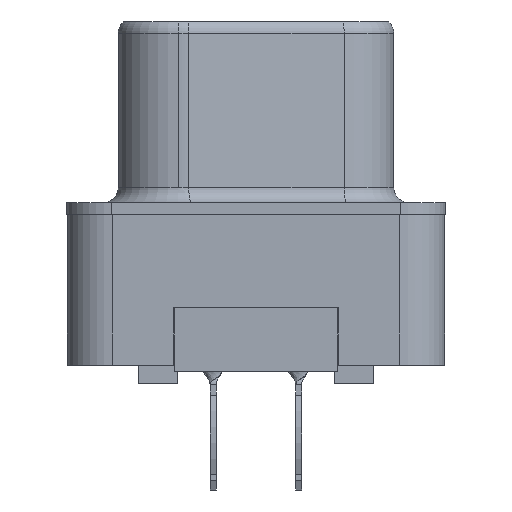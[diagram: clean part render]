
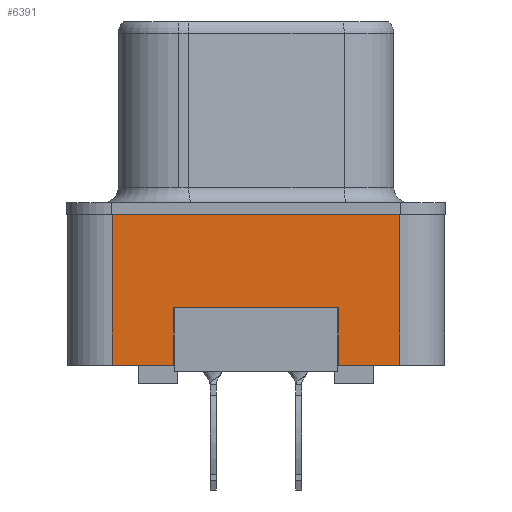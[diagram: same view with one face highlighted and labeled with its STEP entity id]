
A CAD part, left-side view. The second image highlights one B-rep face of the part: STEP entity #6391.
In plain terms, the highlighted planar face has unit normal (-1, 0, 0).
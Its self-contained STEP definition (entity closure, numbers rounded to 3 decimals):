
#1 = ORIENTED_EDGE ( 'NONE', *, *, #18759, .T. ) ;
#488 = CARTESIAN_POINT ( 'NONE',  ( -2.935, 2.75, -5. ) ) ;
#828 = EDGE_CURVE ( 'NONE', #9018, #892, #11236, .T. ) ;
#892 = VERTEX_POINT ( 'NONE', #2387 ) ;
#1121 = CARTESIAN_POINT ( 'NONE',  ( -2.935, -4.775, -5. ) ) ;
#1154 = VECTOR ( 'NONE', #5084, 1000. ) ;
#1344 = LINE ( 'NONE', #2995, #8798 ) ;
#1450 = CARTESIAN_POINT ( 'NONE',  ( -2.935, -4.775, -5. ) ) ;
#2193 = EDGE_CURVE ( 'NONE', #14761, #15495, #1344, .T. ) ;
#2387 = CARTESIAN_POINT ( 'NONE',  ( -2.935, 4.775, 0. ) ) ;
#2432 = VERTEX_POINT ( 'NONE', #14412 ) ;
#2576 = LINE ( 'NONE', #9143, #11425 ) ;
#2875 = DIRECTION ( 'NONE',  ( 0., 1., 0. ) ) ;
#2928 = CARTESIAN_POINT ( 'NONE',  ( -2.935, 2.75, -3.1 ) ) ;
#2995 = CARTESIAN_POINT ( 'NONE',  ( -2.935, -4.775, -5. ) ) ;
#3341 = VECTOR ( 'NONE', #9404, 1000. ) ;
#3846 = ORIENTED_EDGE ( 'NONE', *, *, #14048, .F. ) ;
#3902 = LINE ( 'NONE', #10172, #10526 ) ;
#4223 = DIRECTION ( 'NONE',  ( 0., 0., 1. ) ) ;
#4432 = ORIENTED_EDGE ( 'NONE', *, *, #2193, .T. ) ;
#4819 = VECTOR ( 'NONE', #14530, 1000. ) ;
#4969 = EDGE_CURVE ( 'NONE', #2432, #7586, #2576, .T. ) ;
#5084 = DIRECTION ( 'NONE',  ( 0., 0., -1. ) ) ;
#6235 = CARTESIAN_POINT ( 'NONE',  ( -2.935, -4.775, -5. ) ) ;
#6391 = ADVANCED_FACE ( 'NONE', ( #12022 ), #18310, .T. ) ;
#6490 = DIRECTION ( 'NONE',  ( 0., -1., 0. ) ) ;
#6662 = VECTOR ( 'NONE', #6490, 1000. ) ;
#7586 = VERTEX_POINT ( 'NONE', #2928 ) ;
#7973 = LINE ( 'NONE', #6235, #3341 ) ;
#8088 = DIRECTION ( 'NONE',  ( 0., 0., -1. ) ) ;
#8456 = CARTESIAN_POINT ( 'NONE',  ( -2.935, 4.775, -5. ) ) ;
#8798 = VECTOR ( 'NONE', #15646, 1000. ) ;
#8806 = VERTEX_POINT ( 'NONE', #11970 ) ;
#9018 = VERTEX_POINT ( 'NONE', #12283 ) ;
#9143 = CARTESIAN_POINT ( 'NONE',  ( -2.935, 2.75, -3.1 ) ) ;
#9404 = DIRECTION ( 'NONE',  ( 0., -1., 0. ) ) ;
#9705 = LINE ( 'NONE', #19181, #1154 ) ;
#10050 = VERTEX_POINT ( 'NONE', #488 ) ;
#10172 = CARTESIAN_POINT ( 'NONE',  ( -2.935, -4.775, -5. ) ) ;
#10439 = EDGE_CURVE ( 'NONE', #2432, #8806, #9705, .T. ) ;
#10526 = VECTOR ( 'NONE', #16463, 1000. ) ;
#10897 = ORIENTED_EDGE ( 'NONE', *, *, #4969, .F. ) ;
#10899 = LINE ( 'NONE', #15643, #6662 ) ;
#11236 = LINE ( 'NONE', #8456, #4819 ) ;
#11425 = VECTOR ( 'NONE', #2875, 1000. ) ;
#11970 = CARTESIAN_POINT ( 'NONE',  ( -2.935, -2.75, -5. ) ) ;
#12022 = FACE_OUTER_BOUND ( 'NONE', #12357, .T. ) ;
#12243 = ORIENTED_EDGE ( 'NONE', *, *, #10439, .T. ) ;
#12283 = CARTESIAN_POINT ( 'NONE',  ( -2.935, 4.775, -5. ) ) ;
#12357 = EDGE_LOOP ( 'NONE', ( #12243, #13235, #4432, #12393, #12401, #1, #3846, #10897 ) ) ;
#12393 = ORIENTED_EDGE ( 'NONE', *, *, #19677, .F. ) ;
#12401 = ORIENTED_EDGE ( 'NONE', *, *, #828, .F. ) ;
#13235 = ORIENTED_EDGE ( 'NONE', *, *, #17963, .T. ) ;
#13837 = CARTESIAN_POINT ( 'NONE',  ( -2.935, -4.775, 0. ) ) ;
#13923 = AXIS2_PLACEMENT_3D ( 'NONE', #1121, #16872, #4223 ) ;
#14048 = EDGE_CURVE ( 'NONE', #7586, #10050, #14253, .T. ) ;
#14253 = LINE ( 'NONE', #15905, #16394 ) ;
#14412 = CARTESIAN_POINT ( 'NONE',  ( -2.935, -2.75, -3.1 ) ) ;
#14530 = DIRECTION ( 'NONE',  ( 0., 0., 1. ) ) ;
#14761 = VERTEX_POINT ( 'NONE', #1450 ) ;
#15495 = VERTEX_POINT ( 'NONE', #13837 ) ;
#15643 = CARTESIAN_POINT ( 'NONE',  ( -2.935, -4.775, 0. ) ) ;
#15646 = DIRECTION ( 'NONE',  ( 0., 0., 1. ) ) ;
#15905 = CARTESIAN_POINT ( 'NONE',  ( -2.935, 2.75, -3.1 ) ) ;
#16394 = VECTOR ( 'NONE', #8088, 1000. ) ;
#16463 = DIRECTION ( 'NONE',  ( 0., -1., 0. ) ) ;
#16872 = DIRECTION ( 'NONE',  ( -1., 0., 0. ) ) ;
#17963 = EDGE_CURVE ( 'NONE', #8806, #14761, #3902, .T. ) ;
#18310 = PLANE ( 'NONE',  #13923 ) ;
#18759 = EDGE_CURVE ( 'NONE', #9018, #10050, #7973, .T. ) ;
#19181 = CARTESIAN_POINT ( 'NONE',  ( -2.935, -2.75, -3.1 ) ) ;
#19677 = EDGE_CURVE ( 'NONE', #892, #15495, #10899, .T. ) ;
